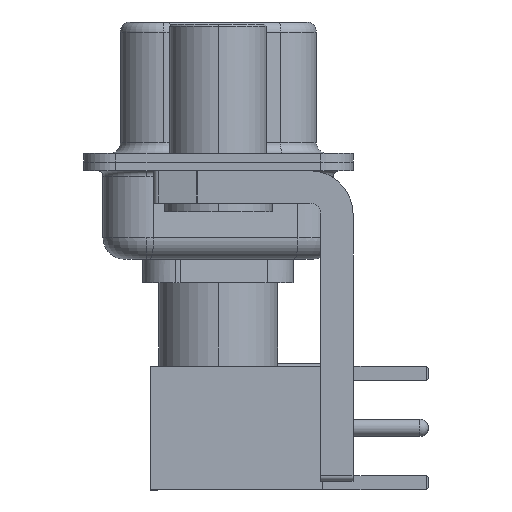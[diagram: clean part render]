
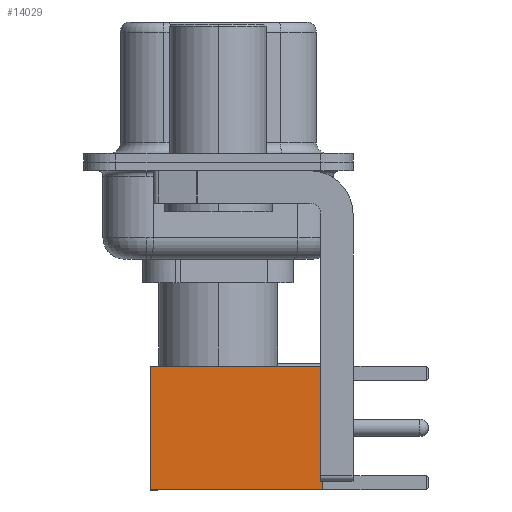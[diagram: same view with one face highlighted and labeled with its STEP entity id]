
A CAD part, left-side view. The second image highlights one B-rep face of the part: STEP entity #14029.
In plain terms, the highlighted face is planar.
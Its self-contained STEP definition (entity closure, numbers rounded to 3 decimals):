
#1788 = LINE ( 'NONE', #28272, #10079 ) ;
#2769 = VERTEX_POINT ( 'NONE', #6969 ) ;
#4076 = DIRECTION ( 'NONE',  ( 0., 0., -1. ) ) ;
#5664 = ORIENTED_EDGE ( 'NONE', *, *, #22507, .F. ) ;
#5919 = VECTOR ( 'NONE', #30345, 1000. ) ;
#6396 = DIRECTION ( 'NONE',  ( 0., 0., 1. ) ) ;
#6969 = CARTESIAN_POINT ( 'NONE',  ( 2.875, 2.875, 8. ) ) ;
#8633 = VECTOR ( 'NONE', #4076, 1000. ) ;
#10079 = VECTOR ( 'NONE', #31304, 1000. ) ;
#11999 = ORIENTED_EDGE ( 'NONE', *, *, #12749, .T. ) ;
#12749 = EDGE_CURVE ( 'NONE', #2769, #15077, #27006, .T. ) ;
#14029 = ADVANCED_FACE ( 'NONE', ( #23334 ), #14051, .T. ) ;
#14051 = PLANE ( 'NONE',  #27237 ) ;
#14725 = CARTESIAN_POINT ( 'NONE',  ( -2.875, 2.875, 0. ) ) ;
#14868 = CARTESIAN_POINT ( 'NONE',  ( 2.875, 2.875, 0. ) ) ;
#15077 = VERTEX_POINT ( 'NONE', #16711 ) ;
#16711 = CARTESIAN_POINT ( 'NONE',  ( 2.875, 2.875, 0. ) ) ;
#17425 = DIRECTION ( 'NONE',  ( 0., 0., -1. ) ) ;
#17518 = EDGE_CURVE ( 'NONE', #2769, #30329, #22729, .T. ) ;
#18685 = DIRECTION ( 'NONE',  ( 0., 1., 0. ) ) ;
#18889 = EDGE_CURVE ( 'NONE', #15077, #25989, #1788, .T. ) ;
#20621 = CARTESIAN_POINT ( 'NONE',  ( 0., 2.875, 8. ) ) ;
#21041 = VECTOR ( 'NONE', #17425, 1000. ) ;
#22507 = EDGE_CURVE ( 'NONE', #30329, #25989, #23244, .T. ) ;
#22729 = LINE ( 'NONE', #20621, #5919 ) ;
#23244 = LINE ( 'NONE', #25624, #8633 ) ;
#23334 = FACE_OUTER_BOUND ( 'NONE', #26275, .T. ) ;
#23805 = CARTESIAN_POINT ( 'NONE',  ( 2.875, 2.875, 0. ) ) ;
#25520 = ORIENTED_EDGE ( 'NONE', *, *, #18889, .T. ) ;
#25624 = CARTESIAN_POINT ( 'NONE',  ( -2.875, 2.875, 0. ) ) ;
#25989 = VERTEX_POINT ( 'NONE', #14725 ) ;
#26275 = EDGE_LOOP ( 'NONE', ( #11999, #25520, #5664, #30529 ) ) ;
#27006 = LINE ( 'NONE', #14868, #21041 ) ;
#27237 = AXIS2_PLACEMENT_3D ( 'NONE', #23805, #18685, #6396 ) ;
#28272 = CARTESIAN_POINT ( 'NONE',  ( 0., 2.875, 0. ) ) ;
#30329 = VERTEX_POINT ( 'NONE', #30797 ) ;
#30345 = DIRECTION ( 'NONE',  ( -1., 0., 0. ) ) ;
#30529 = ORIENTED_EDGE ( 'NONE', *, *, #17518, .F. ) ;
#30797 = CARTESIAN_POINT ( 'NONE',  ( -2.875, 2.875, 8. ) ) ;
#31304 = DIRECTION ( 'NONE',  ( -1., 0., 0. ) ) ;
